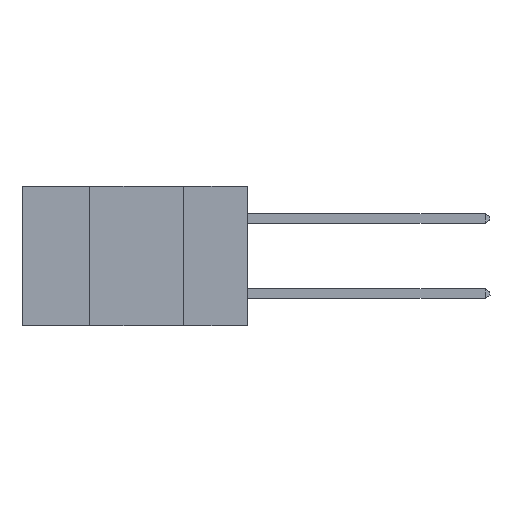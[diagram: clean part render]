
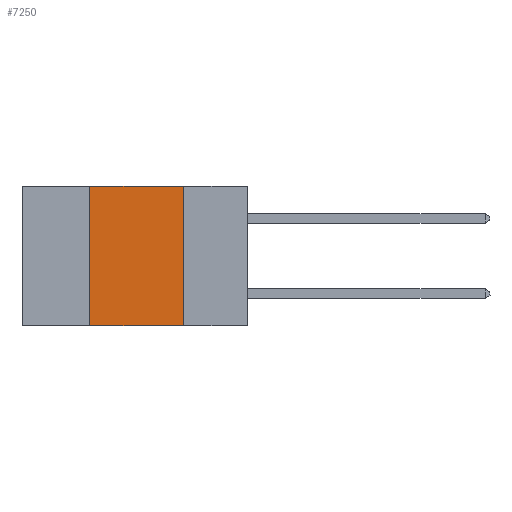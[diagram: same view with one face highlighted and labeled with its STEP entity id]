
A CAD part, left-side view. The second image highlights one B-rep face of the part: STEP entity #7250.
In plain terms, the highlighted planar face has unit normal (-1, 0, 0).
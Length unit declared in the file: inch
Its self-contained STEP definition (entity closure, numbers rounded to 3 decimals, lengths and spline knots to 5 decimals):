
#200 = EDGE_CURVE ( 'NONE', #7938, #4612, #10770, .T. ) ;
#262 = CARTESIAN_POINT ( 'NONE',  ( 0., 0.6, -0.37 ) ) ;
#279 = DIRECTION ( 'NONE',  ( 0., 0., -1. ) ) ;
#382 = LINE ( 'NONE', #262, #8955 ) ;
#502 = CARTESIAN_POINT ( 'NONE',  ( 0., 0.17, 0. ) ) ;
#635 = PLANE ( 'NONE',  #8703 ) ;
#705 = ORIENTED_EDGE ( 'NONE', *, *, #8085, .F. ) ;
#876 = CARTESIAN_POINT ( 'NONE',  ( 0., 0.6, 0. ) ) ;
#902 = VERTEX_POINT ( 'NONE', #8740 ) ;
#1104 = VERTEX_POINT ( 'NONE', #8916 ) ;
#1637 = ORIENTED_EDGE ( 'NONE', *, *, #200, .F. ) ;
#1949 = DIRECTION ( 'NONE',  ( 0., -1., 0. ) ) ;
#1953 = LINE ( 'NONE', #876, #9250 ) ;
#2137 = VECTOR ( 'NONE', #6796, 39.37008 ) ;
#2515 = ORIENTED_EDGE ( 'NONE', *, *, #2617, .T. ) ;
#2617 = EDGE_CURVE ( 'NONE', #902, #4612, #382, .T. ) ;
#3132 = CARTESIAN_POINT ( 'NONE',  ( 0., 0.17, -0.37 ) ) ;
#4158 = DIRECTION ( 'NONE',  ( 1., 0., 0. ) ) ;
#4612 = VERTEX_POINT ( 'NONE', #3132 ) ;
#4958 = EDGE_LOOP ( 'NONE', ( #1637, #705, #9434, #2515 ) ) ;
#5161 = EDGE_CURVE ( 'NONE', #902, #1104, #9308, .T. ) ;
#5743 = DIRECTION ( 'NONE',  ( 0., -1., 0. ) ) ;
#5965 = CARTESIAN_POINT ( 'NONE',  ( 0., 0.42, 0. ) ) ;
#6664 = CARTESIAN_POINT ( 'NONE',  ( 0., 0.6, 0. ) ) ;
#6796 = DIRECTION ( 'NONE',  ( 0., 0., 1. ) ) ;
#7250 = ADVANCED_FACE ( 'NONE', ( #9672 ), #635, .F. ) ;
#7301 = CARTESIAN_POINT ( 'NONE',  ( 0., 0.17, 0. ) ) ;
#7938 = VERTEX_POINT ( 'NONE', #7301 ) ;
#8085 = EDGE_CURVE ( 'NONE', #1104, #7938, #1953, .T. ) ;
#8703 = AXIS2_PLACEMENT_3D ( 'NONE', #6664, #4158, #279 ) ;
#8740 = CARTESIAN_POINT ( 'NONE',  ( 0., 0.42, -0.37 ) ) ;
#8916 = CARTESIAN_POINT ( 'NONE',  ( 0., 0.42, 0. ) ) ;
#8955 = VECTOR ( 'NONE', #1949, 39.37008 ) ;
#9250 = VECTOR ( 'NONE', #5743, 39.37008 ) ;
#9308 = LINE ( 'NONE', #5965, #2137 ) ;
#9434 = ORIENTED_EDGE ( 'NONE', *, *, #5161, .F. ) ;
#9569 = DIRECTION ( 'NONE',  ( 0., 0., -1. ) ) ;
#9672 = FACE_OUTER_BOUND ( 'NONE', #4958, .T. ) ;
#10643 = VECTOR ( 'NONE', #9569, 39.37008 ) ;
#10770 = LINE ( 'NONE', #502, #10643 ) ;
